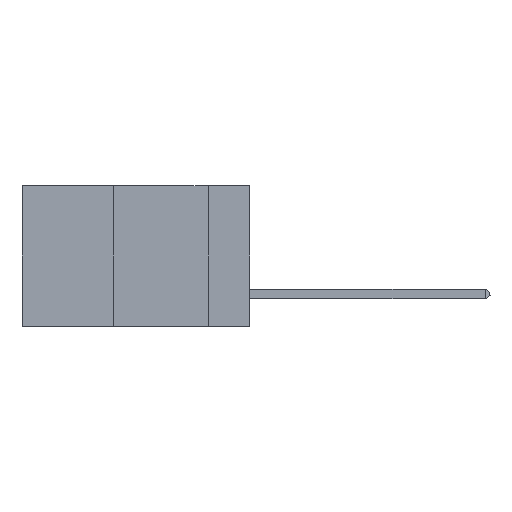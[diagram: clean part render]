
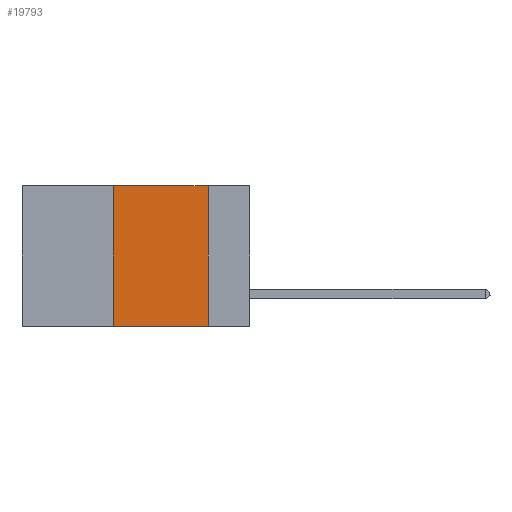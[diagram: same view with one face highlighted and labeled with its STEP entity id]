
A CAD part, left-side view. The second image highlights one B-rep face of the part: STEP entity #19793.
In plain terms, the highlighted planar face has unit normal (-1, 0, 0).
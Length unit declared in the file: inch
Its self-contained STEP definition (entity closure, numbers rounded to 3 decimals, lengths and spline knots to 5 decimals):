
#1050 = CARTESIAN_POINT ( 'NONE',  ( 0., 0.11, 0. ) ) ;
#1367 = EDGE_CURVE ( 'NONE', #10092, #4815, #16528, .T. ) ;
#1912 = DIRECTION ( 'NONE',  ( 0., 0., 1. ) ) ;
#2330 = CARTESIAN_POINT ( 'NONE',  ( 0., 0.6, 0. ) ) ;
#2661 = ORIENTED_EDGE ( 'NONE', *, *, #1367, .T. ) ;
#4267 = EDGE_CURVE ( 'NONE', #6377, #11611, #20651, .T. ) ;
#4815 = VERTEX_POINT ( 'NONE', #14082 ) ;
#6377 = VERTEX_POINT ( 'NONE', #10528 ) ;
#7150 = CARTESIAN_POINT ( 'NONE',  ( 0., 0.6, 0. ) ) ;
#7506 = VECTOR ( 'NONE', #1912, 39.37008 ) ;
#7638 = VECTOR ( 'NONE', #18090, 39.37008 ) ;
#8009 = EDGE_CURVE ( 'NONE', #10092, #6377, #17215, .T. ) ;
#8749 = DIRECTION ( 'NONE',  ( 0., 0., -1. ) ) ;
#9614 = ORIENTED_EDGE ( 'NONE', *, *, #8009, .F. ) ;
#10092 = VERTEX_POINT ( 'NONE', #16836 ) ;
#10440 = DIRECTION ( 'NONE',  ( 0., -1., 0. ) ) ;
#10528 = CARTESIAN_POINT ( 'NONE',  ( 0., 0.36, 0. ) ) ;
#11611 = VERTEX_POINT ( 'NONE', #1050 ) ;
#11743 = CARTESIAN_POINT ( 'NONE',  ( 0., 0.36, 0. ) ) ;
#12482 = ORIENTED_EDGE ( 'NONE', *, *, #4267, .F. ) ;
#12746 = EDGE_LOOP ( 'NONE', ( #13128, #12482, #9614, #2661 ) ) ;
#12928 = VECTOR ( 'NONE', #17884, 39.37008 ) ;
#13128 = ORIENTED_EDGE ( 'NONE', *, *, #19012, .F. ) ;
#13735 = FACE_OUTER_BOUND ( 'NONE', #12746, .T. ) ;
#14082 = CARTESIAN_POINT ( 'NONE',  ( 0., 0.11, -0.37 ) ) ;
#14329 = VECTOR ( 'NONE', #10440, 39.37008 ) ;
#16379 = CARTESIAN_POINT ( 'NONE',  ( 0., 0.6, -0.37 ) ) ;
#16458 = CARTESIAN_POINT ( 'NONE',  ( 0., 0.11, 0. ) ) ;
#16528 = LINE ( 'NONE', #16379, #12928 ) ;
#16836 = CARTESIAN_POINT ( 'NONE',  ( 0., 0.36, -0.37 ) ) ;
#16890 = PLANE ( 'NONE',  #18160 ) ;
#17215 = LINE ( 'NONE', #11743, #7506 ) ;
#17884 = DIRECTION ( 'NONE',  ( 0., -1., 0. ) ) ;
#18090 = DIRECTION ( 'NONE',  ( 0., 0., -1. ) ) ;
#18160 = AXIS2_PLACEMENT_3D ( 'NONE', #2330, #20191, #8749 ) ;
#19012 = EDGE_CURVE ( 'NONE', #11611, #4815, #20096, .T. ) ;
#19793 = ADVANCED_FACE ( 'NONE', ( #13735 ), #16890, .F. ) ;
#20096 = LINE ( 'NONE', #16458, #7638 ) ;
#20191 = DIRECTION ( 'NONE',  ( 1., 0., 0. ) ) ;
#20651 = LINE ( 'NONE', #7150, #14329 ) ;
